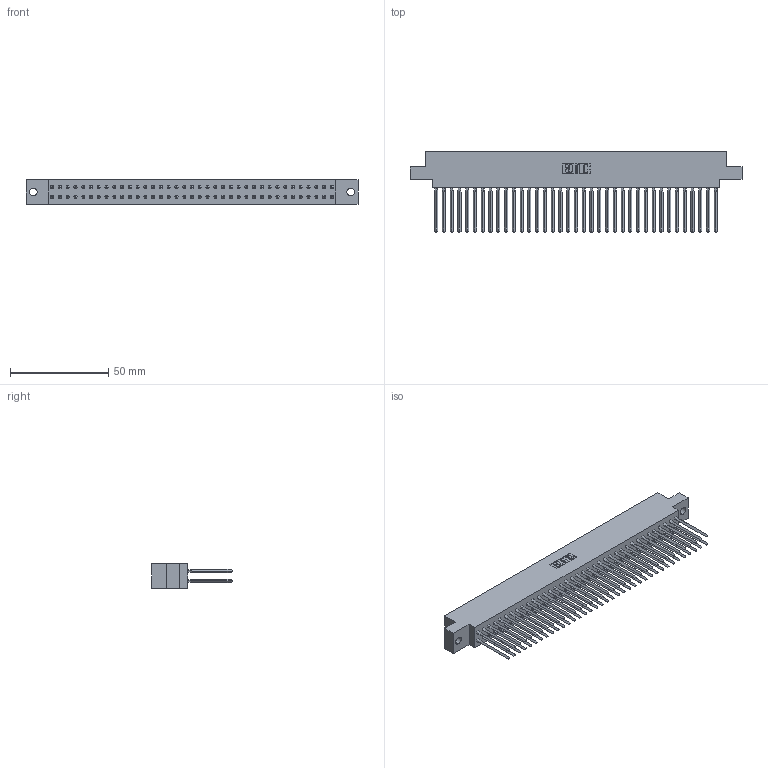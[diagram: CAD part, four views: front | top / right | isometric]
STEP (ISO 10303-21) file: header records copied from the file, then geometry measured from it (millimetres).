
FILE_DESCRIPTION (( 'STEP AP203' ), '1' );
FILE_NAME ('317-074-543-804.STEP', '2020-02-28T08:07:05', ( '' ), ( '' ), 'SwSTEP 2.0', 'SolidWorks 2016', '' );
FILE_SCHEMA (( 'CONFIG_CONTROL_DESIGN' ));
Length unit declared in the file: inch
Products named in the file (3): 317-074-543-804; 317 Part_.156 Dia - TH; 317-290-001_543
Assembly tree (75 placements, depth 2):
  317-074-543-804
    317 Part_.156 Dia - TH
    317-290-001_543  x74
Bounding box: 169.32 x 41.15 x 12.7 mm (x, y, z)
Volume: 28527.9 mm3; surface area: 42908.7 mm2
Topology: 75 solids, 75 shells, 6688 faces, 18553 edges, 11948 vertices
Faces by surface type: plane 5460, cylinder 932, bspline 296
Entity records: 54184 total; most frequent: CARTESIAN_POINT 9867, ORIENTED_EDGE 9366, DIRECTION 7813, EDGE_CURVE 4683, VECTOR 4427, LINE 4427, VERTEX_POINT 3115, AXIS2_PLACEMENT_3D 1693
